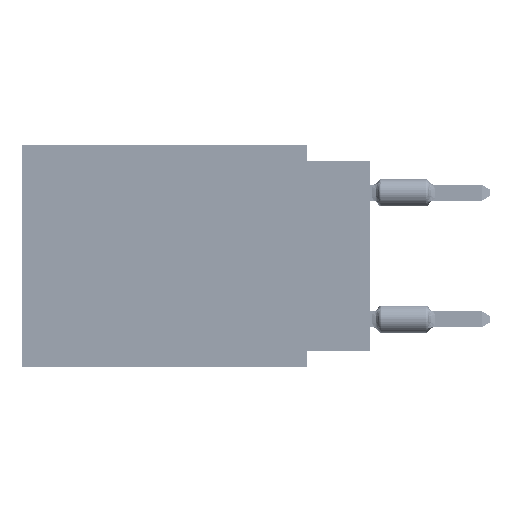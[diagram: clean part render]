
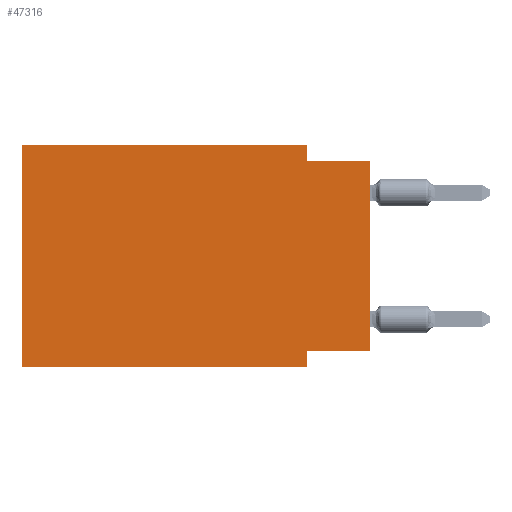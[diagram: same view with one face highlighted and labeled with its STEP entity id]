
A CAD part, left-side view. The second image highlights one B-rep face of the part: STEP entity #47316.
In plain terms, the highlighted planar face has unit normal (-1, 0, 0).
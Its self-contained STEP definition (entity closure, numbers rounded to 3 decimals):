
#1669 = PLANE ( 'NONE',  #56650 ) ;
#3031 = CARTESIAN_POINT ( 'NONE',  ( 0., 2.54, 0. ) ) ;
#3290 = CARTESIAN_POINT ( 'NONE',  ( 0., 0., 0. ) ) ;
#3548 = VECTOR ( 'NONE', #42503, 1000. ) ;
#3639 = LINE ( 'NONE', #3290, #18946 ) ;
#3986 = VECTOR ( 'NONE', #64797, 1000. ) ;
#4342 = ORIENTED_EDGE ( 'NONE', *, *, #34231, .F. ) ;
#4787 = LINE ( 'NONE', #10528, #3548 ) ;
#5106 = VECTOR ( 'NONE', #35379, 1000. ) ;
#5514 = DIRECTION ( 'NONE',  ( 0., -1., 0. ) ) ;
#8255 = VECTOR ( 'NONE', #18165, 1000. ) ;
#8397 = CARTESIAN_POINT ( 'NONE',  ( 0., 2.54, -0.635 ) ) ;
#9565 = EDGE_CURVE ( 'NONE', #13330, #54444, #4787, .T. ) ;
#9699 = CARTESIAN_POINT ( 'NONE',  ( 0., 2.54, 0. ) ) ;
#9837 = CARTESIAN_POINT ( 'NONE',  ( 0., 13.97, -8.89 ) ) ;
#10528 = CARTESIAN_POINT ( 'NONE',  ( 0., 2.54, -8.89 ) ) ;
#11292 = LINE ( 'NONE', #69843, #3986 ) ;
#12302 = EDGE_CURVE ( 'NONE', #15261, #55353, #61255, .T. ) ;
#13330 = VERTEX_POINT ( 'NONE', #61665 ) ;
#13377 = DIRECTION ( 'NONE',  ( 0., 0., 1. ) ) ;
#14974 = CARTESIAN_POINT ( 'NONE',  ( 0., 0., -0.635 ) ) ;
#15146 = EDGE_CURVE ( 'NONE', #53460, #54444, #27060, .T. ) ;
#15261 = VERTEX_POINT ( 'NONE', #66547 ) ;
#15476 = EDGE_CURVE ( 'NONE', #50492, #33939, #3639, .T. ) ;
#16194 = DIRECTION ( 'NONE',  ( 0., -1., 0. ) ) ;
#17278 = ORIENTED_EDGE ( 'NONE', *, *, #15146, .T. ) ;
#18165 = DIRECTION ( 'NONE',  ( 0., -1., 0. ) ) ;
#18946 = VECTOR ( 'NONE', #13377, 1000. ) ;
#19093 = DIRECTION ( 'NONE',  ( 0., 1., 0. ) ) ;
#23581 = CARTESIAN_POINT ( 'NONE',  ( 0., 13.97, 0. ) ) ;
#26936 = VECTOR ( 'NONE', #5514, 1000. ) ;
#27060 = LINE ( 'NONE', #9837, #26936 ) ;
#27923 = VECTOR ( 'NONE', #16194, 1000. ) ;
#30746 = DIRECTION ( 'NONE',  ( 1., 0., 0. ) ) ;
#33939 = VERTEX_POINT ( 'NONE', #14974 ) ;
#33995 = CARTESIAN_POINT ( 'NONE',  ( 0., 0., -8.255 ) ) ;
#34231 = EDGE_CURVE ( 'NONE', #55353, #58608, #46136, .T. ) ;
#34855 = EDGE_CURVE ( 'NONE', #58608, #33939, #48525, .T. ) ;
#35379 = DIRECTION ( 'NONE',  ( 0., 0., -1. ) ) ;
#40271 = ORIENTED_EDGE ( 'NONE', *, *, #34855, .F. ) ;
#42503 = DIRECTION ( 'NONE',  ( 0., 0., -1. ) ) ;
#42820 = ORIENTED_EDGE ( 'NONE', *, *, #54625, .F. ) ;
#44960 = ORIENTED_EDGE ( 'NONE', *, *, #9565, .F. ) ;
#46136 = LINE ( 'NONE', #3031, #5106 ) ;
#46154 = CARTESIAN_POINT ( 'NONE',  ( 0., 2.54, -8.89 ) ) ;
#46858 = CARTESIAN_POINT ( 'NONE',  ( 0., 13.97, 0. ) ) ;
#47077 = LINE ( 'NONE', #68291, #50487 ) ;
#47316 = ADVANCED_FACE ( 'NONE', ( #66683 ), #1669, .F. ) ;
#48525 = LINE ( 'NONE', #59643, #27923 ) ;
#50290 = ORIENTED_EDGE ( 'NONE', *, *, #70298, .F. ) ;
#50487 = VECTOR ( 'NONE', #19093, 1000. ) ;
#50492 = VERTEX_POINT ( 'NONE', #33995 ) ;
#50757 = CARTESIAN_POINT ( 'NONE',  ( 0., 13.97, -8.89 ) ) ;
#52640 = DIRECTION ( 'NONE',  ( 0., 0., -1. ) ) ;
#53460 = VERTEX_POINT ( 'NONE', #50757 ) ;
#54444 = VERTEX_POINT ( 'NONE', #46154 ) ;
#54625 = EDGE_CURVE ( 'NONE', #53460, #15261, #11292, .T. ) ;
#55353 = VERTEX_POINT ( 'NONE', #9699 ) ;
#56650 = AXIS2_PLACEMENT_3D ( 'NONE', #23581, #30746, #52640 ) ;
#58608 = VERTEX_POINT ( 'NONE', #8397 ) ;
#59571 = ORIENTED_EDGE ( 'NONE', *, *, #15476, .T. ) ;
#59643 = CARTESIAN_POINT ( 'NONE',  ( 0., 0., -0.635 ) ) ;
#61255 = LINE ( 'NONE', #46858, #8255 ) ;
#61665 = CARTESIAN_POINT ( 'NONE',  ( 0., 2.54, -8.255 ) ) ;
#61894 = EDGE_LOOP ( 'NONE', ( #59571, #40271, #4342, #67115, #42820, #17278, #44960, #50290 ) ) ;
#64797 = DIRECTION ( 'NONE',  ( 0., 0., 1. ) ) ;
#66547 = CARTESIAN_POINT ( 'NONE',  ( 0., 13.97, 0. ) ) ;
#66683 = FACE_OUTER_BOUND ( 'NONE', #61894, .T. ) ;
#67115 = ORIENTED_EDGE ( 'NONE', *, *, #12302, .F. ) ;
#68291 = CARTESIAN_POINT ( 'NONE',  ( 0., 0., -8.255 ) ) ;
#69843 = CARTESIAN_POINT ( 'NONE',  ( 0., 13.97, 0. ) ) ;
#70298 = EDGE_CURVE ( 'NONE', #50492, #13330, #47077, .T. ) ;
